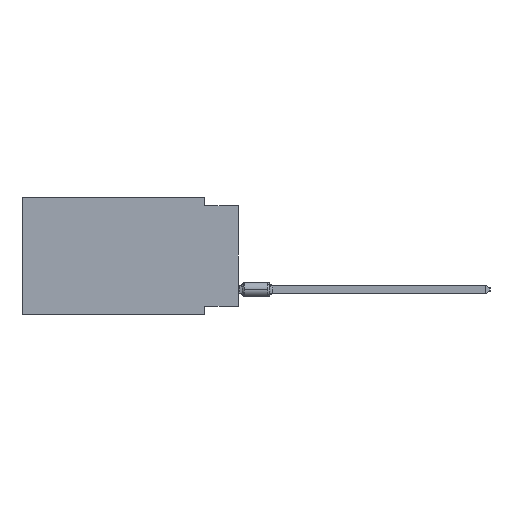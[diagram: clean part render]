
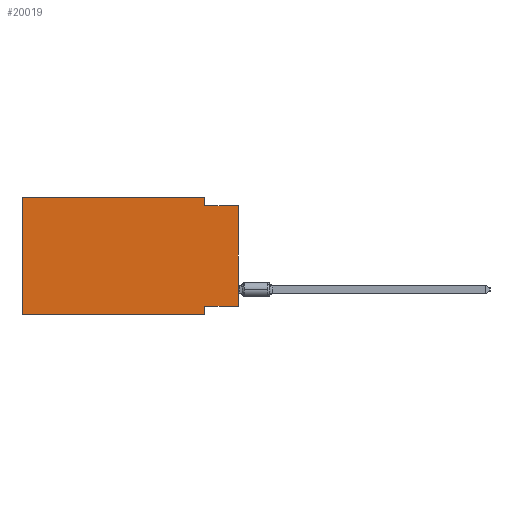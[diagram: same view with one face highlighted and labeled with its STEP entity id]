
A CAD part, left-side view. The second image highlights one B-rep face of the part: STEP entity #20019.
In plain terms, the highlighted planar face has unit normal (-1, 0, 0).
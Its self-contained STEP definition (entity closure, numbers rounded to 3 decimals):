
#352 = PLANE ( 'NONE',  #4678 ) ;
#1625 = LINE ( 'NONE', #11787, #20018 ) ;
#2135 = EDGE_CURVE ( 'NONE', #25955, #62688, #18696, .T. ) ;
#3117 = VECTOR ( 'NONE', #55647, 1000. ) ;
#4678 = AXIS2_PLACEMENT_3D ( 'NONE', #20347, #15413, #20663 ) ;
#4904 = VERTEX_POINT ( 'NONE', #21612 ) ;
#5880 = DIRECTION ( 'NONE',  ( 0., 0., -1. ) ) ;
#6168 = LINE ( 'NONE', #21267, #22916 ) ;
#6722 = ORIENTED_EDGE ( 'NONE', *, *, #45714, .F. ) ;
#8541 = VECTOR ( 'NONE', #35701, 1000. ) ;
#9972 = EDGE_CURVE ( 'NONE', #23169, #19248, #6168, .T. ) ;
#10687 = VERTEX_POINT ( 'NONE', #35785 ) ;
#11787 = CARTESIAN_POINT ( 'NONE',  ( 0., 2.54, 0. ) ) ;
#12837 = VECTOR ( 'NONE', #53766, 1000. ) ;
#13117 = EDGE_CURVE ( 'NONE', #23169, #44475, #55348, .T. ) ;
#14377 = CARTESIAN_POINT ( 'NONE',  ( 0., 0., -0.635 ) ) ;
#15413 = DIRECTION ( 'NONE',  ( 1., 0., 0. ) ) ;
#18696 = LINE ( 'NONE', #53740, #60438 ) ;
#19248 = VERTEX_POINT ( 'NONE', #37565 ) ;
#20018 = VECTOR ( 'NONE', #5880, 1000. ) ;
#20019 = ADVANCED_FACE ( 'NONE', ( #56025 ), #352, .F. ) ;
#20098 = VECTOR ( 'NONE', #34107, 1000. ) ;
#20347 = CARTESIAN_POINT ( 'NONE',  ( 0., 16.383, 0. ) ) ;
#20409 = VERTEX_POINT ( 'NONE', #46149 ) ;
#20663 = DIRECTION ( 'NONE',  ( 0., 0., -1. ) ) ;
#21267 = CARTESIAN_POINT ( 'NONE',  ( 0., 0., -8.255 ) ) ;
#21612 = CARTESIAN_POINT ( 'NONE',  ( 0., 16.383, -8.89 ) ) ;
#22620 = CARTESIAN_POINT ( 'NONE',  ( 0., 16.383, 0. ) ) ;
#22916 = VECTOR ( 'NONE', #45501, 1000. ) ;
#23021 = CARTESIAN_POINT ( 'NONE',  ( 0., 16.383, 0. ) ) ;
#23067 = ORIENTED_EDGE ( 'NONE', *, *, #46879, .F. ) ;
#23169 = VERTEX_POINT ( 'NONE', #27557 ) ;
#25955 = VERTEX_POINT ( 'NONE', #22620 ) ;
#27557 = CARTESIAN_POINT ( 'NONE',  ( 0., 0., -8.255 ) ) ;
#30458 = DIRECTION ( 'NONE',  ( 0., 0., -1. ) ) ;
#32746 = EDGE_CURVE ( 'NONE', #62688, #20409, #1625, .T. ) ;
#33129 = DIRECTION ( 'NONE',  ( 0., -1., 0. ) ) ;
#33487 = CARTESIAN_POINT ( 'NONE',  ( 0., 16.383, -8.89 ) ) ;
#33519 = CARTESIAN_POINT ( 'NONE',  ( 0., 2.54, 0. ) ) ;
#34107 = DIRECTION ( 'NONE',  ( 0., 0., 1. ) ) ;
#35701 = DIRECTION ( 'NONE',  ( 0., 0., 1. ) ) ;
#35785 = CARTESIAN_POINT ( 'NONE',  ( 0., 2.54, -8.89 ) ) ;
#36688 = CARTESIAN_POINT ( 'NONE',  ( 0., 0., 0. ) ) ;
#37193 = LINE ( 'NONE', #33487, #12837 ) ;
#37224 = ORIENTED_EDGE ( 'NONE', *, *, #44536, .F. ) ;
#37565 = CARTESIAN_POINT ( 'NONE',  ( 0., 2.54, -8.255 ) ) ;
#40295 = CARTESIAN_POINT ( 'NONE',  ( 0., 2.54, -8.89 ) ) ;
#43018 = ORIENTED_EDGE ( 'NONE', *, *, #48137, .T. ) ;
#44475 = VERTEX_POINT ( 'NONE', #14377 ) ;
#44536 = EDGE_CURVE ( 'NONE', #20409, #44475, #60561, .T. ) ;
#45501 = DIRECTION ( 'NONE',  ( 0., 1., 0. ) ) ;
#45714 = EDGE_CURVE ( 'NONE', #19248, #10687, #49776, .T. ) ;
#46149 = CARTESIAN_POINT ( 'NONE',  ( 0., 2.54, -0.635 ) ) ;
#46879 = EDGE_CURVE ( 'NONE', #4904, #25955, #59318, .T. ) ;
#47865 = ORIENTED_EDGE ( 'NONE', *, *, #13117, .T. ) ;
#48137 = EDGE_CURVE ( 'NONE', #4904, #10687, #37193, .T. ) ;
#49159 = ORIENTED_EDGE ( 'NONE', *, *, #32746, .F. ) ;
#49256 = ORIENTED_EDGE ( 'NONE', *, *, #2135, .F. ) ;
#49776 = LINE ( 'NONE', #40295, #50262 ) ;
#49851 = EDGE_LOOP ( 'NONE', ( #47865, #37224, #49159, #49256, #23067, #43018, #6722, #52473 ) ) ;
#50262 = VECTOR ( 'NONE', #30458, 1000. ) ;
#52473 = ORIENTED_EDGE ( 'NONE', *, *, #9972, .F. ) ;
#53740 = CARTESIAN_POINT ( 'NONE',  ( 0., 16.383, 0. ) ) ;
#53766 = DIRECTION ( 'NONE',  ( 0., -1., 0. ) ) ;
#55348 = LINE ( 'NONE', #36688, #8541 ) ;
#55647 = DIRECTION ( 'NONE',  ( 0., -1., 0. ) ) ;
#56025 = FACE_OUTER_BOUND ( 'NONE', #49851, .T. ) ;
#59318 = LINE ( 'NONE', #23021, #20098 ) ;
#59611 = CARTESIAN_POINT ( 'NONE',  ( 0., 0., -0.635 ) ) ;
#60438 = VECTOR ( 'NONE', #33129, 1000. ) ;
#60561 = LINE ( 'NONE', #59611, #3117 ) ;
#62688 = VERTEX_POINT ( 'NONE', #33519 ) ;
